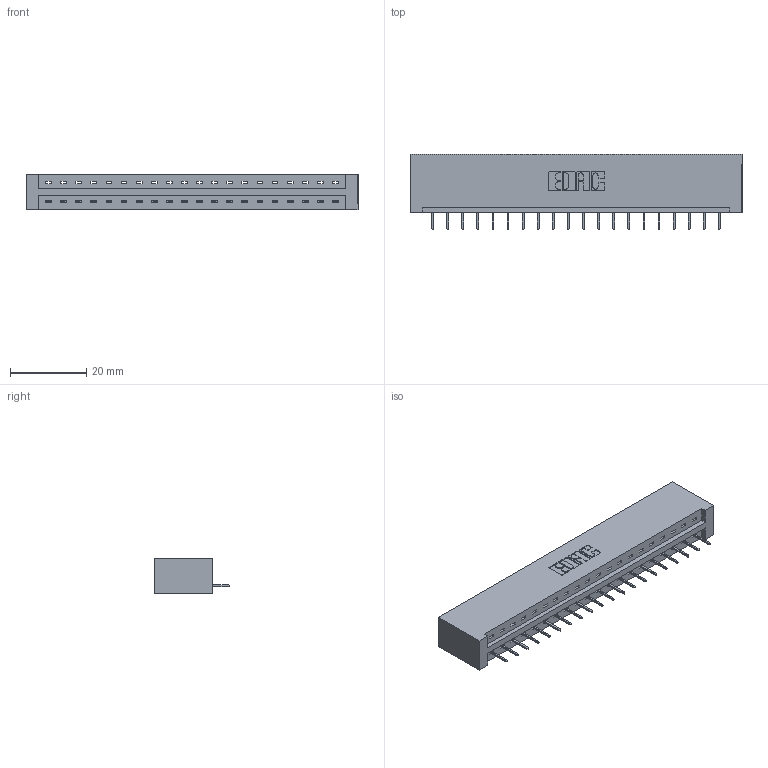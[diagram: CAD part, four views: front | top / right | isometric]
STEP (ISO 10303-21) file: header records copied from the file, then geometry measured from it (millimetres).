
FILE_DESCRIPTION (( 'STEP AP203' ), '1' );
FILE_NAME ('337-020-524-101.STEP', '2019-09-28T22:47:40', ( '' ), ( '' ), 'SwSTEP 2.0', 'SolidWorks 2016', '' );
FILE_SCHEMA (( 'CONFIG_CONTROL_DESIGN' ));
Length unit declared in the file: inch
Products named in the file (3): 337-020-524-101; 337 Part_No Mounting Lugs; 345-292-001_345-293-124
Assembly tree (21 placements, depth 2):
  337-020-524-101
    337 Part_No Mounting Lugs
    345-292-001_345-293-124  x20
Bounding box: 87.12 x 19.69 x 9.4 mm (x, y, z)
Volume: 9439.3 mm3; surface area: 9335.6 mm2
Topology: 21 solids, 21 shells, 1426 faces, 4127 edges, 2670 vertices
Faces by surface type: plane 1106, cylinder 320
Entity records: 17509 total; most frequent: CARTESIAN_POINT 3054, ORIENTED_EDGE 3010, DIRECTION 2609, EDGE_CURVE 1505, LINE 1389, VECTOR 1389, VERTEX_POINT 998, AXIS2_PLACEMENT_3D 610
